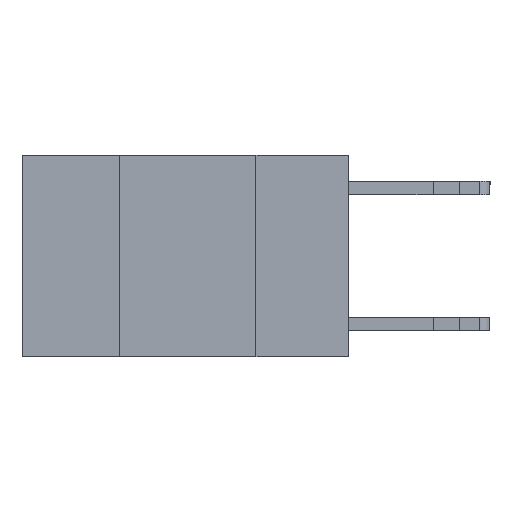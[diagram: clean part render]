
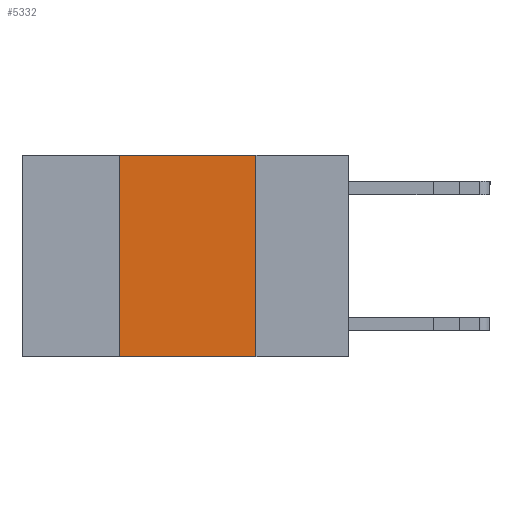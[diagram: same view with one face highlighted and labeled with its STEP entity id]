
A CAD part, left-side view. The second image highlights one B-rep face of the part: STEP entity #5332.
In plain terms, the highlighted planar face has unit normal (-1, 0, 0).
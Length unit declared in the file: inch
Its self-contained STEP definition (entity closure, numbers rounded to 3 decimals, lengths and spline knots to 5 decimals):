
#1166 = CARTESIAN_POINT ( 'NONE',  ( 0., 0.6, 0. ) ) ;
#1557 = VECTOR ( 'NONE', #11799, 39.37008 ) ;
#1589 = CARTESIAN_POINT ( 'NONE',  ( 0., 0.42, 0. ) ) ;
#2088 = LINE ( 'NONE', #2155, #12260 ) ;
#2155 = CARTESIAN_POINT ( 'NONE',  ( 0., 0.6, -0.37 ) ) ;
#2634 = VERTEX_POINT ( 'NONE', #1589 ) ;
#3245 = VERTEX_POINT ( 'NONE', #8636 ) ;
#3589 = EDGE_CURVE ( 'NONE', #7898, #7833, #2088, .T. ) ;
#3737 = EDGE_LOOP ( 'NONE', ( #4191, #9580, #6467, #4256 ) ) ;
#3920 = FACE_OUTER_BOUND ( 'NONE', #3737, .T. ) ;
#3970 = DIRECTION ( 'NONE',  ( 0., 0., -1. ) ) ;
#4060 = VECTOR ( 'NONE', #3970, 39.37008 ) ;
#4191 = ORIENTED_EDGE ( 'NONE', *, *, #7137, .F. ) ;
#4256 = ORIENTED_EDGE ( 'NONE', *, *, #3589, .T. ) ;
#4264 = LINE ( 'NONE', #7239, #6614 ) ;
#5332 = ADVANCED_FACE ( 'NONE', ( #3920 ), #7776, .F. ) ;
#5608 = AXIS2_PLACEMENT_3D ( 'NONE', #1166, #9620, #11530 ) ;
#6371 = EDGE_CURVE ( 'NONE', #2634, #3245, #6918, .T. ) ;
#6467 = ORIENTED_EDGE ( 'NONE', *, *, #10143, .F. ) ;
#6614 = VECTOR ( 'NONE', #8121, 39.37008 ) ;
#6918 = LINE ( 'NONE', #8060, #1557 ) ;
#7016 = DIRECTION ( 'NONE',  ( 0., -1., 0. ) ) ;
#7137 = EDGE_CURVE ( 'NONE', #3245, #7833, #8718, .T. ) ;
#7239 = CARTESIAN_POINT ( 'NONE',  ( 0., 0.42, 0. ) ) ;
#7420 = CARTESIAN_POINT ( 'NONE',  ( 0., 0.17, -0.37 ) ) ;
#7776 = PLANE ( 'NONE',  #5608 ) ;
#7833 = VERTEX_POINT ( 'NONE', #7420 ) ;
#7898 = VERTEX_POINT ( 'NONE', #8323 ) ;
#8060 = CARTESIAN_POINT ( 'NONE',  ( 0., 0.6, 0. ) ) ;
#8121 = DIRECTION ( 'NONE',  ( 0., 0., 1. ) ) ;
#8323 = CARTESIAN_POINT ( 'NONE',  ( 0., 0.42, -0.37 ) ) ;
#8636 = CARTESIAN_POINT ( 'NONE',  ( 0., 0.17, 0. ) ) ;
#8718 = LINE ( 'NONE', #10619, #4060 ) ;
#9580 = ORIENTED_EDGE ( 'NONE', *, *, #6371, .F. ) ;
#9620 = DIRECTION ( 'NONE',  ( 1., 0., 0. ) ) ;
#10143 = EDGE_CURVE ( 'NONE', #7898, #2634, #4264, .T. ) ;
#10619 = CARTESIAN_POINT ( 'NONE',  ( 0., 0.17, 0. ) ) ;
#11530 = DIRECTION ( 'NONE',  ( 0., 0., -1. ) ) ;
#11799 = DIRECTION ( 'NONE',  ( 0., -1., 0. ) ) ;
#12260 = VECTOR ( 'NONE', #7016, 39.37008 ) ;
